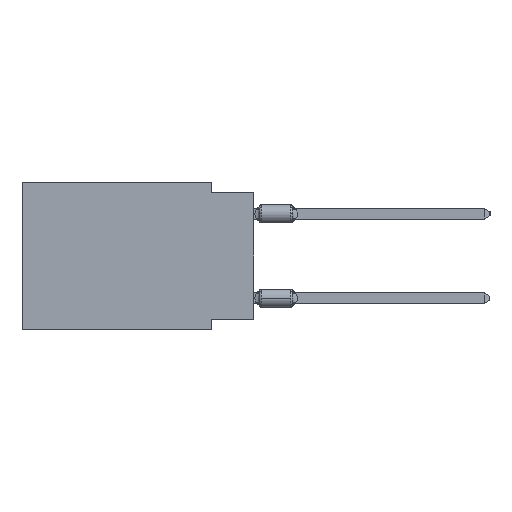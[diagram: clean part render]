
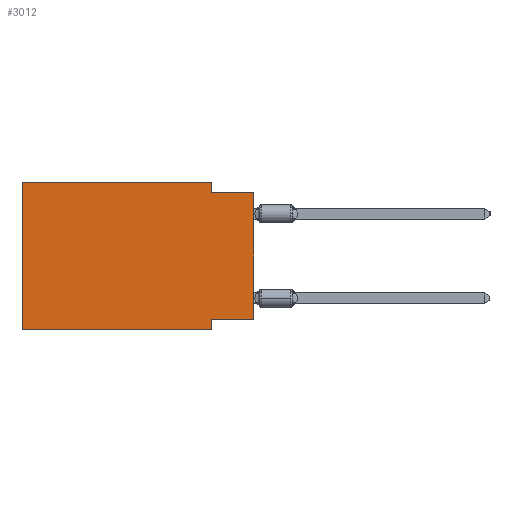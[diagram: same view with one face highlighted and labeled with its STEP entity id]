
A CAD part, left-side view. The second image highlights one B-rep face of the part: STEP entity #3012.
In plain terms, the highlighted planar face has unit normal (-1, 0, 0).
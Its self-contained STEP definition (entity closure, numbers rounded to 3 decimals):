
#541 = CARTESIAN_POINT ( 'NONE',  ( 0., 0., 0. ) ) ;
#1658 = ORIENTED_EDGE ( 'NONE', *, *, #33349, .T. ) ;
#2248 = VECTOR ( 'NONE', #30649, 1000. ) ;
#3012 = ADVANCED_FACE ( 'NONE', ( #25530 ), #6135, .F. ) ;
#3774 = CARTESIAN_POINT ( 'NONE',  ( 0., 0., -0.635 ) ) ;
#3989 = LINE ( 'NONE', #3774, #2248 ) ;
#5324 = ORIENTED_EDGE ( 'NONE', *, *, #38551, .F. ) ;
#6135 = PLANE ( 'NONE',  #19399 ) ;
#10003 = LINE ( 'NONE', #33328, #35325 ) ;
#10495 = LINE ( 'NONE', #10701, #13388 ) ;
#10585 = VECTOR ( 'NONE', #30753, 1000. ) ;
#10701 = CARTESIAN_POINT ( 'NONE',  ( 0., 13.97, -8.89 ) ) ;
#10852 = VECTOR ( 'NONE', #26193, 1000. ) ;
#11169 = CARTESIAN_POINT ( 'NONE',  ( 0., 2.54, 0. ) ) ;
#11206 = VERTEX_POINT ( 'NONE', #43003 ) ;
#11317 = CARTESIAN_POINT ( 'NONE',  ( 0., 13.97, 0. ) ) ;
#12939 = CARTESIAN_POINT ( 'NONE',  ( 0., 2.54, -8.89 ) ) ;
#13388 = VECTOR ( 'NONE', #38213, 1000. ) ;
#13448 = ORIENTED_EDGE ( 'NONE', *, *, #40077, .F. ) ;
#13472 = DIRECTION ( 'NONE',  ( 0., 0., -1. ) ) ;
#14125 = ORIENTED_EDGE ( 'NONE', *, *, #38129, .F. ) ;
#14621 = ORIENTED_EDGE ( 'NONE', *, *, #14883, .F. ) ;
#14780 = VERTEX_POINT ( 'NONE', #22739 ) ;
#14883 = EDGE_CURVE ( 'NONE', #28809, #37037, #3989, .T. ) ;
#17199 = CARTESIAN_POINT ( 'NONE',  ( 0., 2.54, -8.89 ) ) ;
#17317 = LINE ( 'NONE', #11169, #10585 ) ;
#19370 = CARTESIAN_POINT ( 'NONE',  ( 0., 13.97, 0. ) ) ;
#19399 = AXIS2_PLACEMENT_3D ( 'NONE', #42966, #22233, #39633 ) ;
#19598 = VECTOR ( 'NONE', #30273, 1000. ) ;
#20055 = VERTEX_POINT ( 'NONE', #39329 ) ;
#20261 = EDGE_CURVE ( 'NONE', #36679, #20055, #28038, .T. ) ;
#20692 = VECTOR ( 'NONE', #31327, 1000. ) ;
#22206 = CARTESIAN_POINT ( 'NONE',  ( 0., 0., -8.255 ) ) ;
#22233 = DIRECTION ( 'NONE',  ( 1., 0., 0. ) ) ;
#22739 = CARTESIAN_POINT ( 'NONE',  ( 0., 2.54, -8.255 ) ) ;
#23423 = CARTESIAN_POINT ( 'NONE',  ( 0., 13.97, 0. ) ) ;
#23677 = LINE ( 'NONE', #541, #19598 ) ;
#25530 = FACE_OUTER_BOUND ( 'NONE', #43483, .T. ) ;
#25794 = ORIENTED_EDGE ( 'NONE', *, *, #20261, .F. ) ;
#26193 = DIRECTION ( 'NONE',  ( 0., 0., 1. ) ) ;
#28038 = LINE ( 'NONE', #11317, #20692 ) ;
#28648 = LINE ( 'NONE', #19370, #10852 ) ;
#28809 = VERTEX_POINT ( 'NONE', #35651 ) ;
#29148 = EDGE_CURVE ( 'NONE', #20055, #28809, #17317, .T. ) ;
#29720 = VECTOR ( 'NONE', #13472, 1000. ) ;
#30273 = DIRECTION ( 'NONE',  ( 0., 0., 1. ) ) ;
#30649 = DIRECTION ( 'NONE',  ( 0., -1., 0. ) ) ;
#30753 = DIRECTION ( 'NONE',  ( 0., 0., -1. ) ) ;
#30839 = VERTEX_POINT ( 'NONE', #12939 ) ;
#31327 = DIRECTION ( 'NONE',  ( 0., -1., 0. ) ) ;
#33328 = CARTESIAN_POINT ( 'NONE',  ( 0., 0., -8.255 ) ) ;
#33349 = EDGE_CURVE ( 'NONE', #42704, #37037, #23677, .T. ) ;
#33722 = LINE ( 'NONE', #17199, #29720 ) ;
#35246 = EDGE_CURVE ( 'NONE', #11206, #30839, #10495, .T. ) ;
#35325 = VECTOR ( 'NONE', #37514, 1000. ) ;
#35651 = CARTESIAN_POINT ( 'NONE',  ( 0., 2.54, -0.635 ) ) ;
#36679 = VERTEX_POINT ( 'NONE', #23423 ) ;
#37037 = VERTEX_POINT ( 'NONE', #37724 ) ;
#37514 = DIRECTION ( 'NONE',  ( 0., 1., 0. ) ) ;
#37724 = CARTESIAN_POINT ( 'NONE',  ( 0., 0., -0.635 ) ) ;
#38129 = EDGE_CURVE ( 'NONE', #42704, #14780, #10003, .T. ) ;
#38213 = DIRECTION ( 'NONE',  ( 0., -1., 0. ) ) ;
#38551 = EDGE_CURVE ( 'NONE', #14780, #30839, #33722, .T. ) ;
#38784 = ORIENTED_EDGE ( 'NONE', *, *, #35246, .T. ) ;
#39329 = CARTESIAN_POINT ( 'NONE',  ( 0., 2.54, 0. ) ) ;
#39633 = DIRECTION ( 'NONE',  ( 0., 0., -1. ) ) ;
#40077 = EDGE_CURVE ( 'NONE', #11206, #36679, #28648, .T. ) ;
#42489 = ORIENTED_EDGE ( 'NONE', *, *, #29148, .F. ) ;
#42704 = VERTEX_POINT ( 'NONE', #22206 ) ;
#42966 = CARTESIAN_POINT ( 'NONE',  ( 0., 13.97, 0. ) ) ;
#43003 = CARTESIAN_POINT ( 'NONE',  ( 0., 13.97, -8.89 ) ) ;
#43483 = EDGE_LOOP ( 'NONE', ( #1658, #14621, #42489, #25794, #13448, #38784, #5324, #14125 ) ) ;
